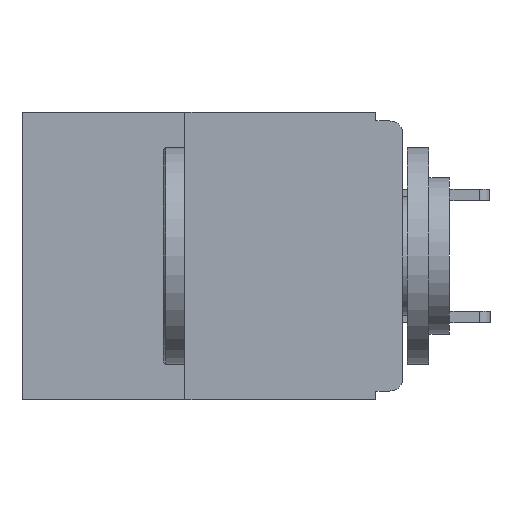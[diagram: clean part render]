
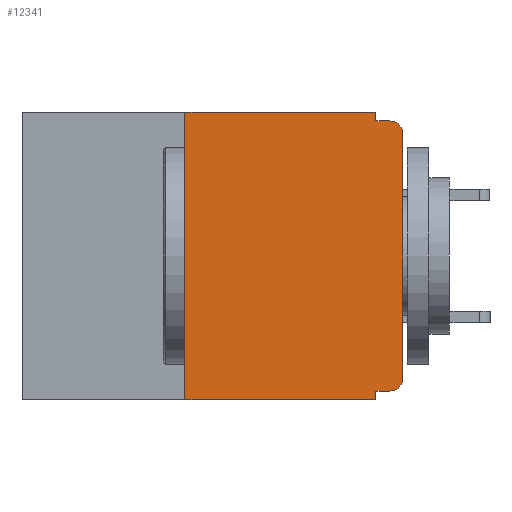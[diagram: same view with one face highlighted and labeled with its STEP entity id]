
A CAD part, left-side view. The second image highlights one B-rep face of the part: STEP entity #12341.
In plain terms, the highlighted planar face has unit normal (-1, 0, 0).
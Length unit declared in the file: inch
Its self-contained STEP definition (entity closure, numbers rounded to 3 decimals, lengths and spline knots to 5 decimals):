
#346 = LINE ( 'NONE', #9249, #13198 ) ;
#382 = VERTEX_POINT ( 'NONE', #30305 ) ;
#576 = DIRECTION ( 'NONE',  ( 0., -1., 0. ) ) ;
#864 = CARTESIAN_POINT ( 'NONE',  ( 0., 0., -0.01 ) ) ;
#1617 = VERTEX_POINT ( 'NONE', #9715 ) ;
#1732 = CARTESIAN_POINT ( 'NONE',  ( 0., 0., 0. ) ) ;
#2986 = CARTESIAN_POINT ( 'NONE',  ( 0., 0.031, -0.33 ) ) ;
#3305 = LINE ( 'NONE', #864, #29276 ) ;
#4423 = CARTESIAN_POINT ( 'NONE',  ( 0., 0.031, -0.33 ) ) ;
#4673 = CARTESIAN_POINT ( 'NONE',  ( 0., 0.25, 0. ) ) ;
#4736 = CARTESIAN_POINT ( 'NONE',  ( 0., 0.437, 0. ) ) ;
#4756 = CARTESIAN_POINT ( 'NONE',  ( 0., 0.015, -0.305 ) ) ;
#5082 = VERTEX_POINT ( 'NONE', #4673 ) ;
#6416 = LINE ( 'NONE', #20757, #18206 ) ;
#6449 = EDGE_CURVE ( 'NONE', #5082, #7315, #346, .T. ) ;
#6986 = AXIS2_PLACEMENT_3D ( 'NONE', #4736, #32255, #17475 ) ;
#7066 = CARTESIAN_POINT ( 'NONE',  ( 0., 0.015, -0.01 ) ) ;
#7315 = VERTEX_POINT ( 'NONE', #9875 ) ;
#7317 = VERTEX_POINT ( 'NONE', #9836 ) ;
#7383 = DIRECTION ( 'NONE',  ( 0., 0., -1. ) ) ;
#8437 = EDGE_CURVE ( 'NONE', #9481, #5082, #6416, .T. ) ;
#8625 = DIRECTION ( 'NONE',  ( 0., -1., 0. ) ) ;
#8755 = LINE ( 'NONE', #28451, #20479 ) ;
#9239 = EDGE_CURVE ( 'NONE', #1617, #7317, #8755, .T. ) ;
#9249 = CARTESIAN_POINT ( 'NONE',  ( 0., 0.437, 0. ) ) ;
#9481 = VERTEX_POINT ( 'NONE', #27020 ) ;
#9715 = CARTESIAN_POINT ( 'NONE',  ( 0., 0.015, -0.32 ) ) ;
#9836 = CARTESIAN_POINT ( 'NONE',  ( 0., 0.031, -0.32 ) ) ;
#9875 = CARTESIAN_POINT ( 'NONE',  ( 0., 0.031, 0. ) ) ;
#11414 = EDGE_CURVE ( 'NONE', #1617, #382, #30033, .T. ) ;
#11733 = VERTEX_POINT ( 'NONE', #28415 ) ;
#11747 = VECTOR ( 'NONE', #576, 39.37008 ) ;
#12341 = ADVANCED_FACE ( 'NONE', ( #16017 ), #27332, .F. ) ;
#12602 = CARTESIAN_POINT ( 'NONE',  ( 0., 0.015, -0.025 ) ) ;
#13198 = VECTOR ( 'NONE', #8625, 39.37008 ) ;
#13620 = EDGE_CURVE ( 'NONE', #11733, #25524, #26396, .T. ) ;
#13720 = DIRECTION ( 'NONE',  ( 0., 1., 0. ) ) ;
#14498 = DIRECTION ( 'NONE',  ( 0., 0., 1. ) ) ;
#15125 = DIRECTION ( 'NONE',  ( 0., 0., -1. ) ) ;
#15856 = CARTESIAN_POINT ( 'NONE',  ( 0., 0.437, -0.33 ) ) ;
#15888 = CARTESIAN_POINT ( 'NONE',  ( 0., 0.031, 0. ) ) ;
#16017 = FACE_OUTER_BOUND ( 'NONE', #29975, .T. ) ;
#16450 = VECTOR ( 'NONE', #23393, 39.37008 ) ;
#17475 = DIRECTION ( 'NONE',  ( 0., 0., -1. ) ) ;
#17525 = VECTOR ( 'NONE', #18202, 39.37008 ) ;
#17946 = AXIS2_PLACEMENT_3D ( 'NONE', #12602, #29954, #15125 ) ;
#18202 = DIRECTION ( 'NONE',  ( 0., 0., -1. ) ) ;
#18206 = VECTOR ( 'NONE', #19832, 39.37008 ) ;
#18336 = LINE ( 'NONE', #15856, #11747 ) ;
#18600 = VECTOR ( 'NONE', #14498, 39.37008 ) ;
#19377 = LINE ( 'NONE', #1732, #18600 ) ;
#19832 = DIRECTION ( 'NONE',  ( 0., 0., 1. ) ) ;
#20391 = ORIENTED_EDGE ( 'NONE', *, *, #32194, .T. ) ;
#20479 = VECTOR ( 'NONE', #13720, 39.37008 ) ;
#20668 = ORIENTED_EDGE ( 'NONE', *, *, #13620, .T. ) ;
#20757 = CARTESIAN_POINT ( 'NONE',  ( 0., 0.25, -0.33 ) ) ;
#20889 = VERTEX_POINT ( 'NONE', #31588 ) ;
#21014 = ORIENTED_EDGE ( 'NONE', *, *, #29504, .F. ) ;
#21599 = ORIENTED_EDGE ( 'NONE', *, *, #30080, .F. ) ;
#21891 = ORIENTED_EDGE ( 'NONE', *, *, #6449, .F. ) ;
#22270 = ORIENTED_EDGE ( 'NONE', *, *, #8437, .F. ) ;
#22299 = ORIENTED_EDGE ( 'NONE', *, *, #25813, .T. ) ;
#22403 = DIRECTION ( 'NONE',  ( -1., 0., 0. ) ) ;
#22589 = LINE ( 'NONE', #2986, #17525 ) ;
#22918 = AXIS2_PLACEMENT_3D ( 'NONE', #4756, #22403, #7383 ) ;
#22933 = ORIENTED_EDGE ( 'NONE', *, *, #31182, .F. ) ;
#23044 = LINE ( 'NONE', #15888, #16450 ) ;
#23340 = ORIENTED_EDGE ( 'NONE', *, *, #9239, .F. ) ;
#23382 = VERTEX_POINT ( 'NONE', #4423 ) ;
#23393 = DIRECTION ( 'NONE',  ( 0., 0., -1. ) ) ;
#23567 = ORIENTED_EDGE ( 'NONE', *, *, #11414, .T. ) ;
#23650 = DIRECTION ( 'NONE',  ( 0., -1., 0. ) ) ;
#25524 = VERTEX_POINT ( 'NONE', #7066 ) ;
#25813 = EDGE_CURVE ( 'NONE', #9481, #23382, #18336, .T. ) ;
#26396 = CIRCLE ( 'NONE', #17946, 0.015 ) ;
#27020 = CARTESIAN_POINT ( 'NONE',  ( 0., 0.25, -0.33 ) ) ;
#27332 = PLANE ( 'NONE',  #6986 ) ;
#28415 = CARTESIAN_POINT ( 'NONE',  ( 0., 0., -0.025 ) ) ;
#28451 = CARTESIAN_POINT ( 'NONE',  ( 0., 0., -0.32 ) ) ;
#29276 = VECTOR ( 'NONE', #23650, 39.37008 ) ;
#29504 = EDGE_CURVE ( 'NONE', #20889, #25524, #3305, .T. ) ;
#29954 = DIRECTION ( 'NONE',  ( -1., 0., 0. ) ) ;
#29975 = EDGE_LOOP ( 'NONE', ( #20391, #20668, #21014, #21599, #21891, #22270, #22299, #22933, #23340, #23567 ) ) ;
#30033 = CIRCLE ( 'NONE', #22918, 0.015 ) ;
#30080 = EDGE_CURVE ( 'NONE', #7315, #20889, #23044, .T. ) ;
#30305 = CARTESIAN_POINT ( 'NONE',  ( 0., 0., -0.305 ) ) ;
#31182 = EDGE_CURVE ( 'NONE', #7317, #23382, #22589, .T. ) ;
#31588 = CARTESIAN_POINT ( 'NONE',  ( 0., 0.031, -0.01 ) ) ;
#32194 = EDGE_CURVE ( 'NONE', #382, #11733, #19377, .T. ) ;
#32255 = DIRECTION ( 'NONE',  ( 1., 0., 0. ) ) ;
